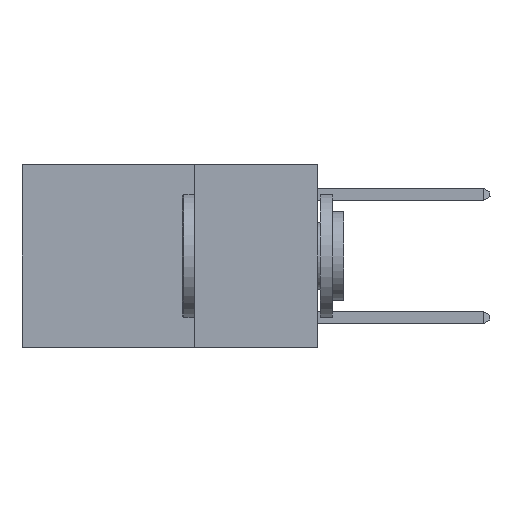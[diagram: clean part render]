
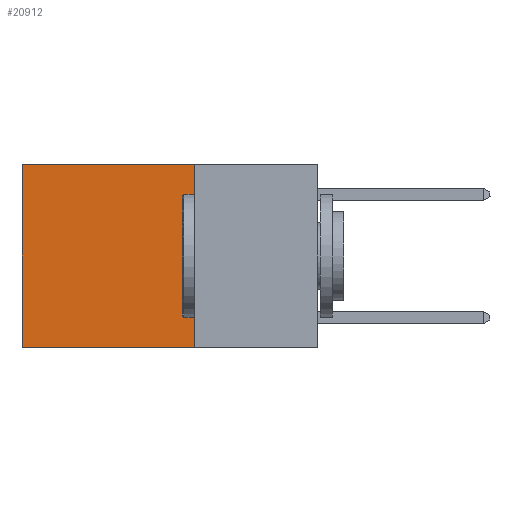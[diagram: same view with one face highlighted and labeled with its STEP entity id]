
A CAD part, left-side view. The second image highlights one B-rep face of the part: STEP entity #20912.
In plain terms, the highlighted planar face has unit normal (-1, 0, 0).
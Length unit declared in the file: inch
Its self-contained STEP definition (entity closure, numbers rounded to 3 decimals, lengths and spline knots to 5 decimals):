
#301 = CARTESIAN_POINT ( 'NONE',  ( 0.2625, 0.25, -0.37 ) ) ;
#878 = VERTEX_POINT ( 'NONE', #2939 ) ;
#1918 = CARTESIAN_POINT ( 'NONE',  ( 0.2625, 0.6, -0.37 ) ) ;
#2939 = CARTESIAN_POINT ( 'NONE',  ( 0.2625, 0.25, 0. ) ) ;
#3871 = PLANE ( 'NONE',  #19354 ) ;
#5120 = CARTESIAN_POINT ( 'NONE',  ( 0.2625, 0.25, 0. ) ) ;
#5526 = VERTEX_POINT ( 'NONE', #1918 ) ;
#5605 = ORIENTED_EDGE ( 'NONE', *, *, #22084, .T. ) ;
#5857 = CARTESIAN_POINT ( 'NONE',  ( 0.2625, 0.25, 0. ) ) ;
#7362 = LINE ( 'NONE', #5120, #23047 ) ;
#8922 = CARTESIAN_POINT ( 'NONE',  ( 0.2625, 0.6, 0. ) ) ;
#10159 = DIRECTION ( 'NONE',  ( 1., 0., 0. ) ) ;
#10390 = ORIENTED_EDGE ( 'NONE', *, *, #15911, .T. ) ;
#11762 = DIRECTION ( 'NONE',  ( 0., 0., -1. ) ) ;
#12133 = LINE ( 'NONE', #18807, #16936 ) ;
#13242 = DIRECTION ( 'NONE',  ( 0., 1., 0. ) ) ;
#13253 = EDGE_LOOP ( 'NONE', ( #5605, #16318, #20396, #10390 ) ) ;
#13605 = LINE ( 'NONE', #17109, #21864 ) ;
#13871 = DIRECTION ( 'NONE',  ( 0., 0., -1. ) ) ;
#14088 = LINE ( 'NONE', #23326, #15031 ) ;
#15031 = VECTOR ( 'NONE', #13242, 39.37008 ) ;
#15773 = DIRECTION ( 'NONE',  ( 0., 1., 0. ) ) ;
#15911 = EDGE_CURVE ( 'NONE', #878, #24991, #13605, .T. ) ;
#16318 = ORIENTED_EDGE ( 'NONE', *, *, #24989, .F. ) ;
#16936 = VECTOR ( 'NONE', #18890, 39.37008 ) ;
#17109 = CARTESIAN_POINT ( 'NONE',  ( 0.2625, 0.25, 0. ) ) ;
#18807 = CARTESIAN_POINT ( 'NONE',  ( 0.2625, 0.6, 0. ) ) ;
#18890 = DIRECTION ( 'NONE',  ( 0., 0., -1. ) ) ;
#19354 = AXIS2_PLACEMENT_3D ( 'NONE', #5857, #10159, #13871 ) ;
#20396 = ORIENTED_EDGE ( 'NONE', *, *, #20993, .F. ) ;
#20912 = ADVANCED_FACE ( 'NONE', ( #24395 ), #3871, .F. ) ;
#20993 = EDGE_CURVE ( 'NONE', #878, #23040, #7362, .T. ) ;
#21864 = VECTOR ( 'NONE', #15773, 39.37008 ) ;
#22084 = EDGE_CURVE ( 'NONE', #24991, #5526, #12133, .T. ) ;
#23040 = VERTEX_POINT ( 'NONE', #301 ) ;
#23047 = VECTOR ( 'NONE', #11762, 39.37008 ) ;
#23326 = CARTESIAN_POINT ( 'NONE',  ( 0.2625, 0.25, -0.37 ) ) ;
#24395 = FACE_OUTER_BOUND ( 'NONE', #13253, .T. ) ;
#24989 = EDGE_CURVE ( 'NONE', #23040, #5526, #14088, .T. ) ;
#24991 = VERTEX_POINT ( 'NONE', #8922 ) ;
